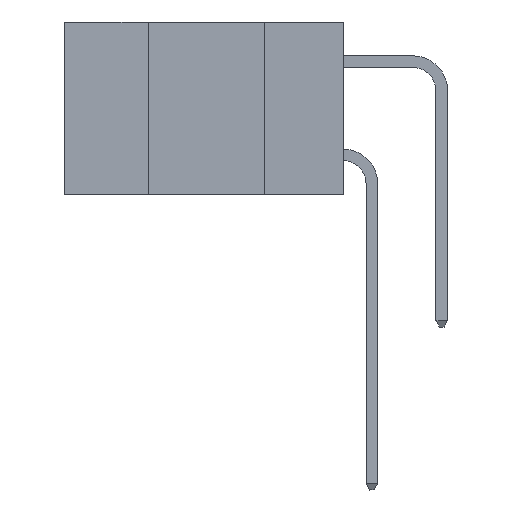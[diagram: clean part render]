
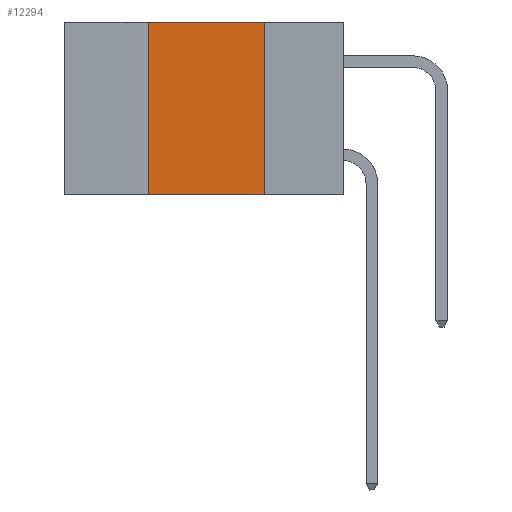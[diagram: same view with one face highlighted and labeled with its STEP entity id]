
A CAD part, left-side view. The second image highlights one B-rep face of the part: STEP entity #12294.
In plain terms, the highlighted planar face has unit normal (-1, 0, 0).
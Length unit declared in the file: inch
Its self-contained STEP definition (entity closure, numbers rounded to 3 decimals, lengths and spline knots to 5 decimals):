
#1074 = DIRECTION ( 'NONE',  ( 0., -1., 0. ) ) ;
#1446 = ORIENTED_EDGE ( 'NONE', *, *, #10701, .F. ) ;
#1576 = VERTEX_POINT ( 'NONE', #9332 ) ;
#1605 = DIRECTION ( 'NONE',  ( 1., 0., 0. ) ) ;
#2971 = CARTESIAN_POINT ( 'NONE',  ( 0., 0.17, 0. ) ) ;
#3003 = LINE ( 'NONE', #7821, #8904 ) ;
#5298 = VECTOR ( 'NONE', #1074, 39.37008 ) ;
#6008 = LINE ( 'NONE', #18716, #5298 ) ;
#6635 = VERTEX_POINT ( 'NONE', #2971 ) ;
#7356 = ORIENTED_EDGE ( 'NONE', *, *, #12160, .F. ) ;
#7821 = CARTESIAN_POINT ( 'NONE',  ( 0., 0.42, -0.37 ) ) ;
#8067 = ORIENTED_EDGE ( 'NONE', *, *, #13606, .T. ) ;
#8510 = AXIS2_PLACEMENT_3D ( 'NONE', #21332, #1605, #17045 ) ;
#8693 = LINE ( 'NONE', #18843, #13808 ) ;
#8904 = VECTOR ( 'NONE', #16572, 39.37008 ) ;
#9332 = CARTESIAN_POINT ( 'NONE',  ( 0., 0.17, -0.37 ) ) ;
#10094 = VERTEX_POINT ( 'NONE', #18186 ) ;
#10609 = FACE_OUTER_BOUND ( 'NONE', #26933, .T. ) ;
#10701 = EDGE_CURVE ( 'NONE', #27510, #6635, #12080, .T. ) ;
#12080 = LINE ( 'NONE', #19960, #16546 ) ;
#12160 = EDGE_CURVE ( 'NONE', #10094, #27510, #3003, .T. ) ;
#12294 = ADVANCED_FACE ( 'NONE', ( #10609 ), #27902, .F. ) ;
#13606 = EDGE_CURVE ( 'NONE', #10094, #1576, #6008, .T. ) ;
#13808 = VECTOR ( 'NONE', #23345, 39.37008 ) ;
#16546 = VECTOR ( 'NONE', #22171, 39.37008 ) ;
#16572 = DIRECTION ( 'NONE',  ( 0., 0., 1. ) ) ;
#17002 = ORIENTED_EDGE ( 'NONE', *, *, #24954, .F. ) ;
#17045 = DIRECTION ( 'NONE',  ( 0., 0., -1. ) ) ;
#18186 = CARTESIAN_POINT ( 'NONE',  ( 0., 0.42, -0.37 ) ) ;
#18716 = CARTESIAN_POINT ( 'NONE',  ( 0., 0.6, -0.37 ) ) ;
#18843 = CARTESIAN_POINT ( 'NONE',  ( 0., 0.17, -0.37 ) ) ;
#19960 = CARTESIAN_POINT ( 'NONE',  ( 0., 0.6, 0. ) ) ;
#21332 = CARTESIAN_POINT ( 'NONE',  ( 0., 0.6, 0. ) ) ;
#22171 = DIRECTION ( 'NONE',  ( 0., -1., 0. ) ) ;
#23345 = DIRECTION ( 'NONE',  ( 0., 0., -1. ) ) ;
#24954 = EDGE_CURVE ( 'NONE', #6635, #1576, #8693, .T. ) ;
#25587 = CARTESIAN_POINT ( 'NONE',  ( 0., 0.42, 0. ) ) ;
#26933 = EDGE_LOOP ( 'NONE', ( #17002, #1446, #7356, #8067 ) ) ;
#27510 = VERTEX_POINT ( 'NONE', #25587 ) ;
#27902 = PLANE ( 'NONE',  #8510 ) ;
